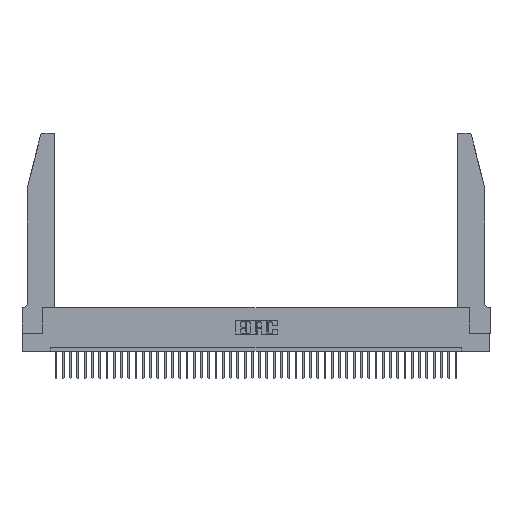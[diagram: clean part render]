
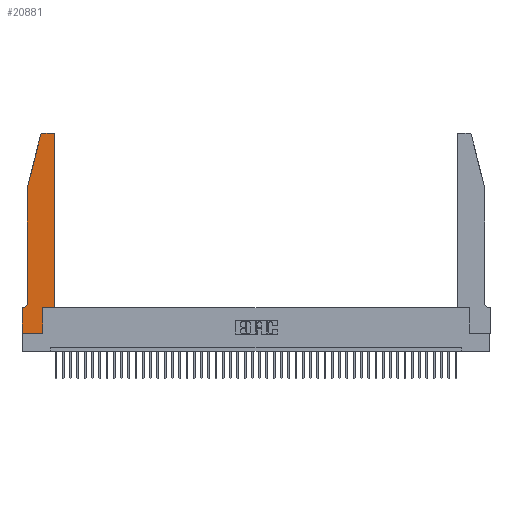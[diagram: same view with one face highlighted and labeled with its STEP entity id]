
A CAD part, top view. The second image highlights one B-rep face of the part: STEP entity #20881.
In plain terms, the highlighted planar face has unit normal (0, 0, 1).
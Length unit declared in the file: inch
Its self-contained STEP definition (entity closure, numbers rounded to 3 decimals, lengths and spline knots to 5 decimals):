
#464 = VERTEX_POINT ( 'NONE', #16960 ) ;
#602 = CARTESIAN_POINT ( 'NONE',  ( 0.284, 2.72, 0.37 ) ) ;
#749 = ORIENTED_EDGE ( 'NONE', *, *, #14137, .T. ) ;
#2256 = LINE ( 'NONE', #9335, #42512 ) ;
#2605 = DIRECTION ( 'NONE',  ( 1., 0., 0. ) ) ;
#2862 = LINE ( 'NONE', #4077, #5019 ) ;
#2930 = PLANE ( 'NONE',  #44660 ) ;
#3465 = DIRECTION ( 'NONE',  ( 0., -1., 0. ) ) ;
#3778 = ORIENTED_EDGE ( 'NONE', *, *, #36203, .T. ) ;
#3794 = CARTESIAN_POINT ( 'NONE',  ( 0., 0.35, 0.37 ) ) ;
#4077 = CARTESIAN_POINT ( 'NONE',  ( 0.0755, 0.35, 0.37 ) ) ;
#4211 = DIRECTION ( 'NONE',  ( 0., 0., 1. ) ) ;
#4287 = VERTEX_POINT ( 'NONE', #29146 ) ;
#5019 = VECTOR ( 'NONE', #28476, 39.37008 ) ;
#5628 = CARTESIAN_POINT ( 'NONE',  ( 0.4505, 0.35, 0.37 ) ) ;
#6068 = VECTOR ( 'NONE', #29303, 39.37008 ) ;
#6359 = ORIENTED_EDGE ( 'NONE', *, *, #20092, .T. ) ;
#7000 = CIRCLE ( 'NONE', #33631, 0.03 ) ;
#7773 = LINE ( 'NONE', #17195, #9482 ) ;
#7926 = VERTEX_POINT ( 'NONE', #39005 ) ;
#8406 = CARTESIAN_POINT ( 'NONE',  ( 0.4505, 0.35, 0.37 ) ) ;
#9335 = CARTESIAN_POINT ( 'NONE',  ( 0.2605, 2.75, 0.37 ) ) ;
#9482 = VECTOR ( 'NONE', #3465, 39.37008 ) ;
#9513 = DIRECTION ( 'NONE',  ( -0.239, -0.971, 0. ) ) ;
#9650 = VECTOR ( 'NONE', #9513, 39.37008 ) ;
#10518 = DIRECTION ( 'NONE',  ( 1., 0., 0. ) ) ;
#10587 = VERTEX_POINT ( 'NONE', #22960 ) ;
#10702 = CARTESIAN_POINT ( 'NONE',  ( 0.25487, 2.72718, 0.37 ) ) ;
#11761 = CARTESIAN_POINT ( 'NONE',  ( 0.0755, 2., 0.37 ) ) ;
#11887 = CIRCLE ( 'NONE', #27813, 0.03 ) ;
#12058 = ORIENTED_EDGE ( 'NONE', *, *, #25279, .T. ) ;
#12262 = CARTESIAN_POINT ( 'NONE',  ( 0.0755, 2., 0.37 ) ) ;
#12987 = ORIENTED_EDGE ( 'NONE', *, *, #43496, .T. ) ;
#13160 = EDGE_CURVE ( 'NONE', #24126, #10587, #39762, .T. ) ;
#13430 = LINE ( 'NONE', #12262, #9650 ) ;
#13550 = EDGE_CURVE ( 'NONE', #7926, #41287, #28874, .T. ) ;
#14137 = EDGE_CURVE ( 'NONE', #4287, #17732, #7000, .T. ) ;
#14687 = CARTESIAN_POINT ( 'NONE',  ( 0., 0., 0.37 ) ) ;
#14708 = DIRECTION ( 'NONE',  ( 1., 0., 0. ) ) ;
#14784 = ORIENTED_EDGE ( 'NONE', *, *, #17759, .T. ) ;
#14796 = ORIENTED_EDGE ( 'NONE', *, *, #25420, .T. ) ;
#15217 = VERTEX_POINT ( 'NONE', #14687 ) ;
#15284 = EDGE_LOOP ( 'NONE', ( #40715, #749, #6359, #43409, #12058, #14796, #12987, #14784, #42772, #44887, #15366, #3778 ) ) ;
#15366 = ORIENTED_EDGE ( 'NONE', *, *, #13550, .T. ) ;
#16104 = VECTOR ( 'NONE', #35046, 39.37008 ) ;
#16263 = VECTOR ( 'NONE', #23152, 39.37008 ) ;
#16279 = CARTESIAN_POINT ( 'NONE',  ( 0.4205, 2.72, 0.37 ) ) ;
#16960 = CARTESIAN_POINT ( 'NONE',  ( 0.0055, 0.35, 0.37 ) ) ;
#16963 = VERTEX_POINT ( 'NONE', #37652 ) ;
#17195 = CARTESIAN_POINT ( 'NONE',  ( 0., 0., 0.37 ) ) ;
#17359 = CARTESIAN_POINT ( 'NONE',  ( 0.2865, 0.35, 0.37 ) ) ;
#17732 = VERTEX_POINT ( 'NONE', #10702 ) ;
#17759 = EDGE_CURVE ( 'NONE', #15217, #39719, #41976, .T. ) ;
#17928 = DIRECTION ( 'NONE',  ( 0., -1., 0. ) ) ;
#18274 = LINE ( 'NONE', #17359, #16104 ) ;
#18436 = LINE ( 'NONE', #5628, #16263 ) ;
#19058 = VERTEX_POINT ( 'NONE', #22013 ) ;
#19337 = DIRECTION ( 'NONE',  ( -1., 0., 0. ) ) ;
#19439 = VERTEX_POINT ( 'NONE', #34359 ) ;
#20092 = EDGE_CURVE ( 'NONE', #17732, #24126, #13430, .T. ) ;
#20881 = ADVANCED_FACE ( 'NONE', ( #33666 ), #2930, .T. ) ;
#22013 = CARTESIAN_POINT ( 'NONE',  ( 0., 0.35, 0.37 ) ) ;
#22960 = CARTESIAN_POINT ( 'NONE',  ( 0.0755, 0.42, 0.37 ) ) ;
#23152 = DIRECTION ( 'NONE',  ( 1., 0., 0. ) ) ;
#23963 = EDGE_CURVE ( 'NONE', #39719, #19439, #18274, .T. ) ;
#24126 = VERTEX_POINT ( 'NONE', #11761 ) ;
#25279 = EDGE_CURVE ( 'NONE', #10587, #464, #31831, .T. ) ;
#25420 = EDGE_CURVE ( 'NONE', #464, #19058, #2862, .T. ) ;
#25768 = CARTESIAN_POINT ( 'NONE',  ( 0.2865, 0., 0.37 ) ) ;
#27235 = VECTOR ( 'NONE', #17928, 39.37008 ) ;
#27314 = CARTESIAN_POINT ( 'NONE',  ( 0.4505, 2.72, 0.37 ) ) ;
#27790 = VECTOR ( 'NONE', #30226, 39.37008 ) ;
#27813 = AXIS2_PLACEMENT_3D ( 'NONE', #16279, #41238, #2605 ) ;
#28476 = DIRECTION ( 'NONE',  ( -1., 0., 0. ) ) ;
#28489 = AXIS2_PLACEMENT_3D ( 'NONE', #32772, #43039, #19337 ) ;
#28874 = LINE ( 'NONE', #8406, #27790 ) ;
#28989 = CARTESIAN_POINT ( 'NONE',  ( 0., 0., 0.37 ) ) ;
#29146 = CARTESIAN_POINT ( 'NONE',  ( 0.284, 2.75, 0.37 ) ) ;
#29303 = DIRECTION ( 'NONE',  ( 1., 0., 0. ) ) ;
#30226 = DIRECTION ( 'NONE',  ( 0., 1., 0. ) ) ;
#31831 = CIRCLE ( 'NONE', #28489, 0.07 ) ;
#31996 = EDGE_CURVE ( 'NONE', #16963, #4287, #2256, .T. ) ;
#32772 = CARTESIAN_POINT ( 'NONE',  ( 0.0055, 0.42, 0.37 ) ) ;
#33631 = AXIS2_PLACEMENT_3D ( 'NONE', #602, #4211, #14708 ) ;
#33666 = FACE_OUTER_BOUND ( 'NONE', #15284, .T. ) ;
#34224 = DIRECTION ( 'NONE',  ( -1., 0., 0. ) ) ;
#34359 = CARTESIAN_POINT ( 'NONE',  ( 0.2865, 0.35, 0.37 ) ) ;
#35046 = DIRECTION ( 'NONE',  ( 0., 1., 0. ) ) ;
#36167 = EDGE_CURVE ( 'NONE', #19439, #7926, #18436, .T. ) ;
#36203 = EDGE_CURVE ( 'NONE', #41287, #16963, #11887, .T. ) ;
#37652 = CARTESIAN_POINT ( 'NONE',  ( 0.4205, 2.75, 0.37 ) ) ;
#39005 = CARTESIAN_POINT ( 'NONE',  ( 0.4505, 0.35, 0.37 ) ) ;
#39719 = VERTEX_POINT ( 'NONE', #25768 ) ;
#39762 = LINE ( 'NONE', #44585, #27235 ) ;
#40715 = ORIENTED_EDGE ( 'NONE', *, *, #31996, .T. ) ;
#41238 = DIRECTION ( 'NONE',  ( 0., 0., 1. ) ) ;
#41287 = VERTEX_POINT ( 'NONE', #27314 ) ;
#41976 = LINE ( 'NONE', #28989, #6068 ) ;
#42166 = DIRECTION ( 'NONE',  ( 0., 0., 1. ) ) ;
#42512 = VECTOR ( 'NONE', #34224, 39.37008 ) ;
#42772 = ORIENTED_EDGE ( 'NONE', *, *, #23963, .T. ) ;
#43039 = DIRECTION ( 'NONE',  ( 0., 0., -1. ) ) ;
#43409 = ORIENTED_EDGE ( 'NONE', *, *, #13160, .T. ) ;
#43496 = EDGE_CURVE ( 'NONE', #19058, #15217, #7773, .T. ) ;
#44585 = CARTESIAN_POINT ( 'NONE',  ( 0.0755, 2., 0.37 ) ) ;
#44660 = AXIS2_PLACEMENT_3D ( 'NONE', #3794, #42166, #10518 ) ;
#44887 = ORIENTED_EDGE ( 'NONE', *, *, #36167, .T. ) ;
